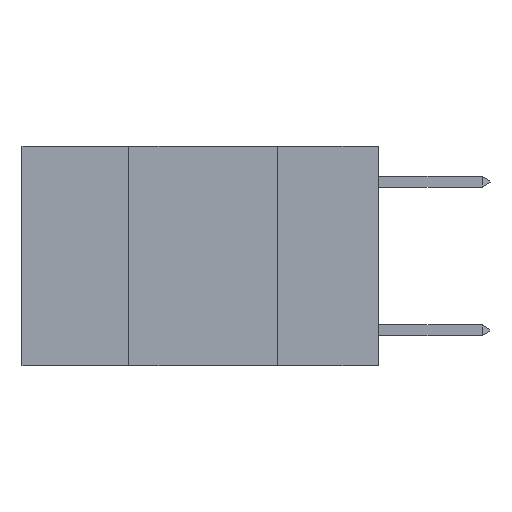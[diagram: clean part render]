
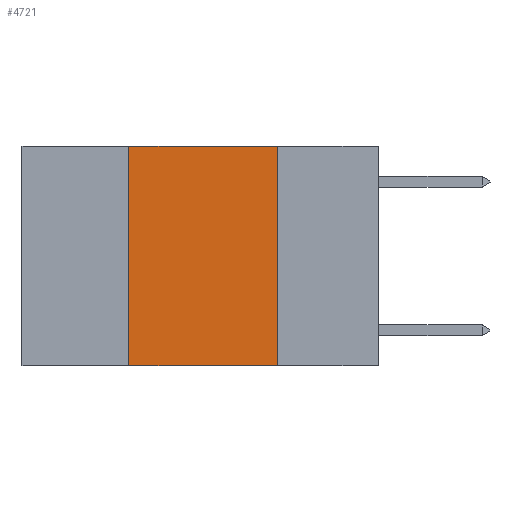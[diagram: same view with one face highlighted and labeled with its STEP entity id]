
A CAD part, left-side view. The second image highlights one B-rep face of the part: STEP entity #4721.
In plain terms, the highlighted planar face has unit normal (-1, 0, 0).
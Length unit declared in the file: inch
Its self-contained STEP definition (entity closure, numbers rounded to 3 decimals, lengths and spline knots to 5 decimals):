
#31 = VECTOR ( 'NONE', #12143, 39.37008 ) ;
#132 = CARTESIAN_POINT ( 'NONE',  ( 0., 0.17, 0. ) ) ;
#322 = AXIS2_PLACEMENT_3D ( 'NONE', #16409, #11406, #1107 ) ;
#356 = CARTESIAN_POINT ( 'NONE',  ( 0., 0.42, 0. ) ) ;
#1107 = DIRECTION ( 'NONE',  ( 0., 0., -1. ) ) ;
#1872 = LINE ( 'NONE', #356, #15004 ) ;
#2819 = LINE ( 'NONE', #18430, #11465 ) ;
#4186 = VERTEX_POINT ( 'NONE', #6274 ) ;
#4233 = ORIENTED_EDGE ( 'NONE', *, *, #6271, .T. ) ;
#4585 = LINE ( 'NONE', #8071, #13239 ) ;
#4721 = ADVANCED_FACE ( 'NONE', ( #5566 ), #21484, .F. ) ;
#5469 = DIRECTION ( 'NONE',  ( 0., 0., 1. ) ) ;
#5566 = FACE_OUTER_BOUND ( 'NONE', #18233, .T. ) ;
#6271 = EDGE_CURVE ( 'NONE', #9728, #10734, #2819, .T. ) ;
#6274 = CARTESIAN_POINT ( 'NONE',  ( 0., 0.42, 0. ) ) ;
#8071 = CARTESIAN_POINT ( 'NONE',  ( 0., 0.6, 0. ) ) ;
#8301 = CARTESIAN_POINT ( 'NONE',  ( 0., 0.42, -0.37 ) ) ;
#8734 = EDGE_CURVE ( 'NONE', #4186, #19412, #4585, .T. ) ;
#9728 = VERTEX_POINT ( 'NONE', #8301 ) ;
#10734 = VERTEX_POINT ( 'NONE', #17820 ) ;
#11406 = DIRECTION ( 'NONE',  ( 1., 0., 0. ) ) ;
#11465 = VECTOR ( 'NONE', #16713, 39.37008 ) ;
#12143 = DIRECTION ( 'NONE',  ( 0., 0., -1. ) ) ;
#12878 = ORIENTED_EDGE ( 'NONE', *, *, #17850, .F. ) ;
#13239 = VECTOR ( 'NONE', #18280, 39.37008 ) ;
#15004 = VECTOR ( 'NONE', #5469, 39.37008 ) ;
#16409 = CARTESIAN_POINT ( 'NONE',  ( 0., 0.6, 0. ) ) ;
#16570 = LINE ( 'NONE', #132, #31 ) ;
#16713 = DIRECTION ( 'NONE',  ( 0., -1., 0. ) ) ;
#16807 = CARTESIAN_POINT ( 'NONE',  ( 0., 0.17, 0. ) ) ;
#17724 = EDGE_CURVE ( 'NONE', #19412, #10734, #16570, .T. ) ;
#17820 = CARTESIAN_POINT ( 'NONE',  ( 0., 0.17, -0.37 ) ) ;
#17850 = EDGE_CURVE ( 'NONE', #9728, #4186, #1872, .T. ) ;
#18233 = EDGE_LOOP ( 'NONE', ( #20758, #21275, #12878, #4233 ) ) ;
#18280 = DIRECTION ( 'NONE',  ( 0., -1., 0. ) ) ;
#18430 = CARTESIAN_POINT ( 'NONE',  ( 0., 0.6, -0.37 ) ) ;
#19412 = VERTEX_POINT ( 'NONE', #16807 ) ;
#20758 = ORIENTED_EDGE ( 'NONE', *, *, #17724, .F. ) ;
#21275 = ORIENTED_EDGE ( 'NONE', *, *, #8734, .F. ) ;
#21484 = PLANE ( 'NONE',  #322 ) ;
